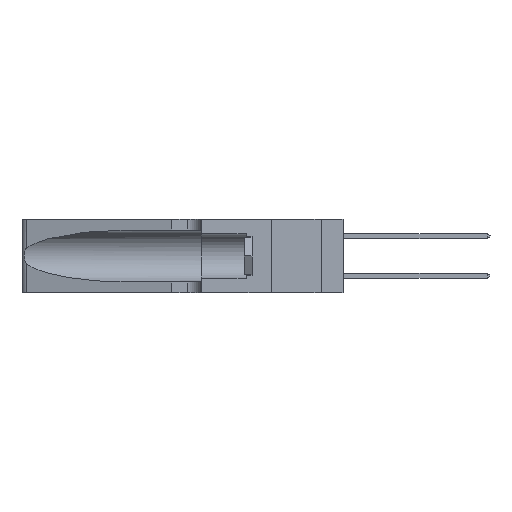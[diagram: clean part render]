
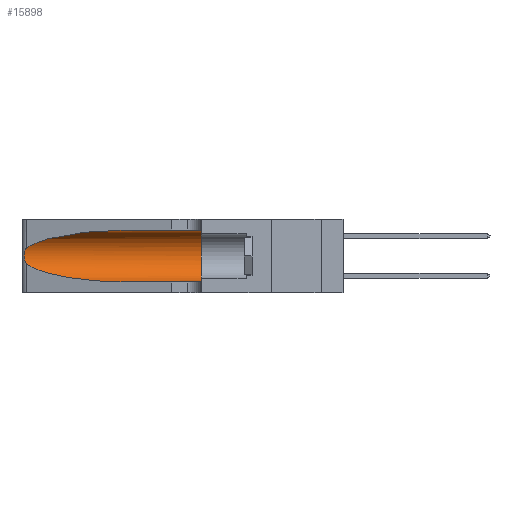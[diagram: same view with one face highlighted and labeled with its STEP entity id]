
A CAD part, left-side view. The second image highlights one B-rep face of the part: STEP entity #15898.
In plain terms, the highlighted cylindrical face has radius 3.308 mm (diameter 6.617 mm), a partial arc.
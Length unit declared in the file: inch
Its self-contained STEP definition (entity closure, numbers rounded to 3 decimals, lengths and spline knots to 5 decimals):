
#662 = LINE ( 'NONE', #5834, #36921 ) ;
#672 = CARTESIAN_POINT ( 'NONE',  ( 0.1305, 0.72297, 0.31525 ) ) ;
#2133 = CARTESIAN_POINT ( 'NONE',  ( 0.25487, 1.22718, 0.22369 ) ) ;
#2283 = EDGE_LOOP ( 'NONE', ( #38445, #33107, #9572, #12754, #17837, #19391 ) ) ;
#2287 = CARTESIAN_POINT ( 'NONE',  ( 0.25639, 1.23186, 0.15144 ) ) ;
#2524 = DIRECTION ( 'NONE',  ( 0., 0., -1. ) ) ;
#3673 = EDGE_CURVE ( 'NONE', #12542, #24774, #25904, .T. ) ;
#5834 = CARTESIAN_POINT ( 'NONE',  ( 0.1305, 1.61858, 0.31525 ) ) ;
#6158 = CARTESIAN_POINT ( 'NONE',  ( 0.25487, 1.22718, 0.14631 ) ) ;
#7109 = CYLINDRICAL_SURFACE ( 'NONE', #38534, 0.13025 ) ;
#7496 = VERTEX_POINT ( 'NONE', #33528 ) ;
#9572 = ORIENTED_EDGE ( 'NONE', *, *, #43084, .T. ) ;
#9802 = CARTESIAN_POINT ( 'NONE',  ( 0.25487, 1.22718, 0.14631 ) ) ;
#9872 = CARTESIAN_POINT ( 'NONE',  ( 0.25639, 1.23184, 0.21858 ) ) ;
#10838 = EDGE_CURVE ( 'NONE', #24774, #24955, #21724, .T. ) ;
#11203 = LINE ( 'NONE', #29447, #29769 ) ;
#12542 = VERTEX_POINT ( 'NONE', #672 ) ;
#12754 = ORIENTED_EDGE ( 'NONE', *, *, #31455, .T. ) ;
#12960 = VERTEX_POINT ( 'NONE', #45115 ) ;
#13257 = DIRECTION ( 'NONE',  ( 0., 1., 0. ) ) ;
#13465 = DIRECTION ( 'NONE',  ( 0., -1., 0. ) ) ;
#13617 = CARTESIAN_POINT ( 'NONE',  ( 0.25854, 1.2359, 0.20912 ) ) ;
#15898 = ADVANCED_FACE ( 'NONE', ( #37975 ), #7109, .F. ) ;
#17102 = EDGE_CURVE ( 'NONE', #12960, #7496, #23940, .T. ) ;
#17337 = CARTESIAN_POINT ( 'NONE',  ( 0.26075, 1.23896, 0.19203 ) ) ;
#17837 = ORIENTED_EDGE ( 'NONE', *, *, #17102, .F. ) ;
#19391 = ORIENTED_EDGE ( 'NONE', *, *, #37087, .F. ) ;
#19847 = CARTESIAN_POINT ( 'NONE',  ( 0.2373, 1.15595, 0.28018 ) ) ;
#20996 = CARTESIAN_POINT ( 'NONE',  ( 0.1305, 0.72297, 0.05475 ) ) ;
#21064 = CARTESIAN_POINT ( 'NONE',  ( 0.26017, 1.23833, 0.17102 ) ) ;
#21724 = B_SPLINE_CURVE_WITH_KNOTS ( 'NONE', 3,
 ( #2133, #24610, #9872, #35813, #13617, #39533, #17337, #43261, #21064, #46956, #24769, #2287, #28533, #6158 ),
 .UNSPECIFIED., .F., .F.,
 ( 4, 2, 2, 2, 2, 2, 4 ),
 ( 0., 0.00027, 0.00053, 0.00107, 0.0016, 0.00187, 0.00214 ),
 .UNSPECIFIED. ) ;
#22380 = AXIS2_PLACEMENT_3D ( 'NONE', #35454, #13257, #39179 ) ;
#23056 = VERTEX_POINT ( 'NONE', #34456 ) ;
#23553 = CARTESIAN_POINT ( 'NONE',  ( 0.1305, 0.72297, 0.31525 ) ) ;
#23940 = CIRCLE ( 'NONE', #22380, 0.13025 ) ;
#24610 = CARTESIAN_POINT ( 'NONE',  ( 0.25555, 1.22994, 0.2215 ) ) ;
#24769 = CARTESIAN_POINT ( 'NONE',  ( 0.25789, 1.23486, 0.15765 ) ) ;
#24774 = VERTEX_POINT ( 'NONE', #25495 ) ;
#24955 = VERTEX_POINT ( 'NONE', #42049 ) ;
#24979 = DIRECTION ( 'NONE',  ( 0., -1., 0. ) ) ;
#25495 = CARTESIAN_POINT ( 'NONE',  ( 0.25487, 1.22718, 0.22369 ) ) ;
#25904 =( BOUNDED_CURVE ( )  B_SPLINE_CURVE ( 3, ( #23553, #45742, #19847, #27315 ),
 .UNSPECIFIED., .F., .F. ) 
 B_SPLINE_CURVE_WITH_KNOTS ( ( 4, 4 ),
 ( 1.5708, 2.84003 ),
 .UNSPECIFIED. ) 
 CURVE ( )  GEOMETRIC_REPRESENTATION_ITEM ( )  RATIONAL_B_SPLINE_CURVE ( ( 1., 0.87, 0.87, 1. ) ) 
 REPRESENTATION_ITEM ( '' )  );
#27315 = CARTESIAN_POINT ( 'NONE',  ( 0.25487, 1.22718, 0.22369 ) ) ;
#28305 = CARTESIAN_POINT ( 'NONE',  ( 0.2373, 1.15595, 0.08982 ) ) ;
#28533 = CARTESIAN_POINT ( 'NONE',  ( 0.25555, 1.22993, 0.14849 ) ) ;
#28753 = CARTESIAN_POINT ( 'NONE',  ( 0.1305, 1.61858, 0.185 ) ) ;
#29447 = CARTESIAN_POINT ( 'NONE',  ( 0.1305, 1.61858, 0.05475 ) ) ;
#29769 = VECTOR ( 'NONE', #33161, 39.37008 ) ;
#31455 = EDGE_CURVE ( 'NONE', #23056, #7496, #11203, .T. ) ;
#31670 =( BOUNDED_CURVE ( )  B_SPLINE_CURVE ( 3, ( #9802, #28305, #43195, #20996 ),
 .UNSPECIFIED., .F., .F. ) 
 B_SPLINE_CURVE_WITH_KNOTS ( ( 4, 4 ),
 ( 3.44316, 4.71239 ),
 .UNSPECIFIED. ) 
 CURVE ( )  GEOMETRIC_REPRESENTATION_ITEM ( )  RATIONAL_B_SPLINE_CURVE ( ( 1., 0.87, 0.87, 1. ) ) 
 REPRESENTATION_ITEM ( '' )  );
#33107 = ORIENTED_EDGE ( 'NONE', *, *, #10838, .T. ) ;
#33161 = DIRECTION ( 'NONE',  ( 0., -1., 0. ) ) ;
#33528 = CARTESIAN_POINT ( 'NONE',  ( 0.1305, 0.35, 0.05475 ) ) ;
#34456 = CARTESIAN_POINT ( 'NONE',  ( 0.1305, 0.72297, 0.05475 ) ) ;
#35454 = CARTESIAN_POINT ( 'NONE',  ( 0.1305, 0.35, 0.185 ) ) ;
#35813 = CARTESIAN_POINT ( 'NONE',  ( 0.25787, 1.23484, 0.2124 ) ) ;
#36921 = VECTOR ( 'NONE', #13465, 39.37008 ) ;
#37087 = EDGE_CURVE ( 'NONE', #12542, #12960, #662, .T. ) ;
#37975 = FACE_OUTER_BOUND ( 'NONE', #2283, .T. ) ;
#38445 = ORIENTED_EDGE ( 'NONE', *, *, #3673, .T. ) ;
#38534 = AXIS2_PLACEMENT_3D ( 'NONE', #28753, #24979, #2524 ) ;
#39179 = DIRECTION ( 'NONE',  ( 0., 0., 1. ) ) ;
#39533 = CARTESIAN_POINT ( 'NONE',  ( 0.26018, 1.23835, 0.19895 ) ) ;
#42049 = CARTESIAN_POINT ( 'NONE',  ( 0.25487, 1.22718, 0.14631 ) ) ;
#43084 = EDGE_CURVE ( 'NONE', #24955, #23056, #31670, .T. ) ;
#43195 = CARTESIAN_POINT ( 'NONE',  ( 0.18966, 0.96281, 0.05475 ) ) ;
#43261 = CARTESIAN_POINT ( 'NONE',  ( 0.26075, 1.23896, 0.178 ) ) ;
#45115 = CARTESIAN_POINT ( 'NONE',  ( 0.1305, 0.35, 0.31525 ) ) ;
#45742 = CARTESIAN_POINT ( 'NONE',  ( 0.18966, 0.96281, 0.31525 ) ) ;
#46956 = CARTESIAN_POINT ( 'NONE',  ( 0.25856, 1.23593, 0.16098 ) ) ;
